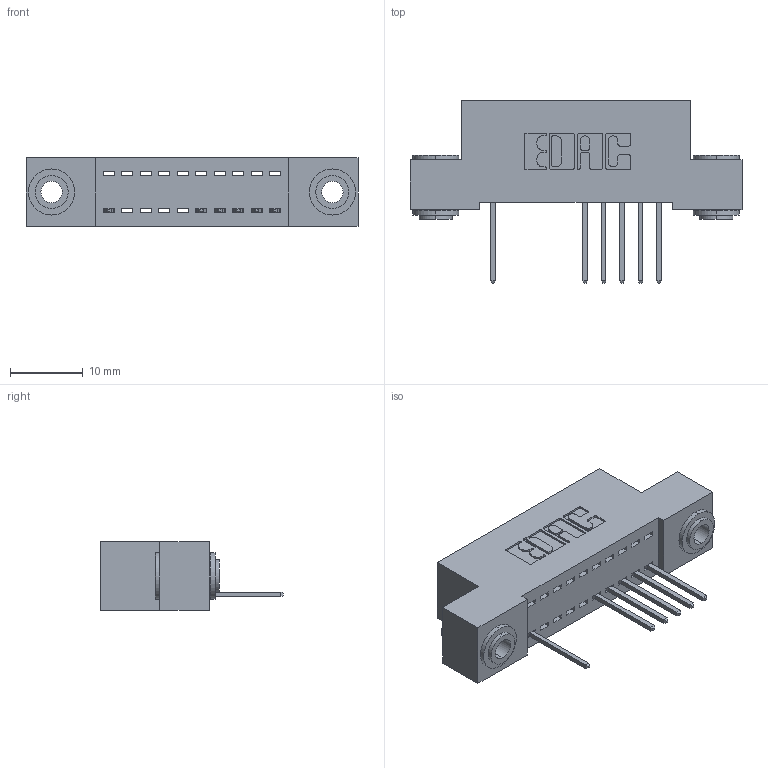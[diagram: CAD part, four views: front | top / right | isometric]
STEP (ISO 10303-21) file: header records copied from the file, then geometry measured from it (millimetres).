
FILE_DESCRIPTION (( 'STEP AP203' ), '1' );
FILE_NAME ('392-010-523-103.STEP', '2018-08-14T20:14:14', ( '' ), ( '' ), 'SwSTEP 2.0', 'SolidWorks 2016', '' );
FILE_SCHEMA (( 'CONFIG_CONTROL_DESIGN' ));
Length unit declared in the file: inch
Products named in the file (4): 342 Part_.156 TH; 345-292-001_345-293-123; 342-250-002_345-250-002-102; 392-010-523-103
Assembly tree (9 placements, depth 2):
  392-010-523-103
    342 Part_.156 TH
    345-292-001_345-293-123  x6
    342-250-002_345-250-002-102  x2
Bounding box: 45.72 x 25.15 x 9.4 mm (x, y, z)
Volume: 3865.6 mm3; surface area: 5073.8 mm2
Topology: 9 solids, 9 shells, 544 faces, 1599 edges, 1054 vertices
Faces by surface type: plane 376, cylinder 160, cone 8
Entity records: 10660 total; most frequent: CARTESIAN_POINT 1839, ORIENTED_EDGE 1782, DIRECTION 1645, EDGE_CURVE 891, LINE 739, VECTOR 739, VERTEX_POINT 590, AXIS2_PLACEMENT_3D 453
